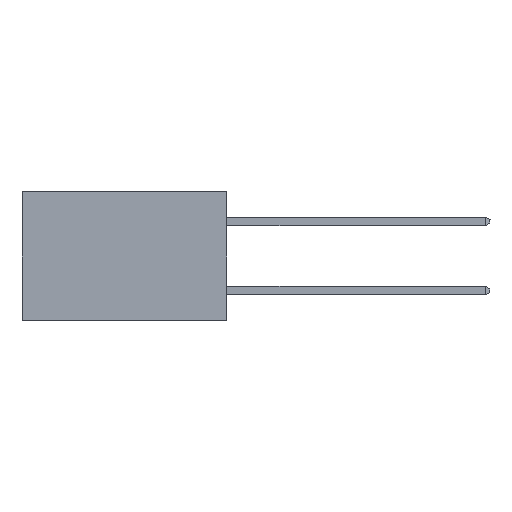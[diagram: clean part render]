
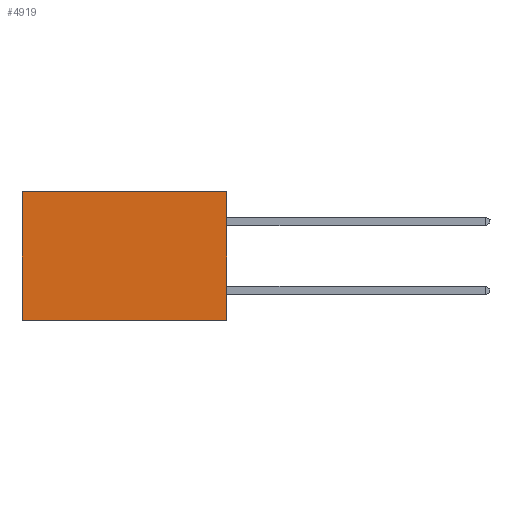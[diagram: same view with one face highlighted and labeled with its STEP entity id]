
A CAD part, left-side view. The second image highlights one B-rep face of the part: STEP entity #4919.
In plain terms, the highlighted planar face has unit normal (-1, 0, 0).
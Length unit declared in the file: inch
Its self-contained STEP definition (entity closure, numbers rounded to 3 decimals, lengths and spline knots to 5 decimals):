
#410 = VECTOR ( 'NONE', #22200, 39.37008 ) ;
#917 = ORIENTED_EDGE ( 'NONE', *, *, #23986, .T. ) ;
#2059 = VECTOR ( 'NONE', #22672, 39.37008 ) ;
#3909 = ORIENTED_EDGE ( 'NONE', *, *, #14130, .F. ) ;
#4919 = ADVANCED_FACE ( 'NONE', ( #15475 ), #14348, .F. ) ;
#5017 = LINE ( 'NONE', #8824, #410 ) ;
#6903 = DIRECTION ( 'NONE',  ( 0., 1., 0. ) ) ;
#8143 = VERTEX_POINT ( 'NONE', #18027 ) ;
#8751 = EDGE_CURVE ( 'NONE', #8143, #22815, #14476, .T. ) ;
#8824 = CARTESIAN_POINT ( 'NONE',  ( 0.277, 0.59, -0.37 ) ) ;
#9307 = VECTOR ( 'NONE', #23433, 39.37008 ) ;
#9668 = EDGE_CURVE ( 'NONE', #15816, #21993, #19501, .T. ) ;
#11166 = EDGE_LOOP ( 'NONE', ( #917, #11948, #3909, #24839 ) ) ;
#11948 = ORIENTED_EDGE ( 'NONE', *, *, #9668, .F. ) ;
#12706 = CARTESIAN_POINT ( 'NONE',  ( 0.277, 0., -0.37 ) ) ;
#12944 = AXIS2_PLACEMENT_3D ( 'NONE', #13612, #13324, #13297 ) ;
#13297 = DIRECTION ( 'NONE',  ( 0., 0., -1. ) ) ;
#13324 = DIRECTION ( 'NONE',  ( 1., 0., 0. ) ) ;
#13612 = CARTESIAN_POINT ( 'NONE',  ( 0.277, 0., -0.37 ) ) ;
#14130 = EDGE_CURVE ( 'NONE', #8143, #15816, #21454, .T. ) ;
#14348 = PLANE ( 'NONE',  #12944 ) ;
#14476 = LINE ( 'NONE', #21560, #9307 ) ;
#14868 = CARTESIAN_POINT ( 'NONE',  ( 0.277, 0.59, 0. ) ) ;
#15475 = FACE_OUTER_BOUND ( 'NONE', #11166, .T. ) ;
#15816 = VERTEX_POINT ( 'NONE', #15846 ) ;
#15846 = CARTESIAN_POINT ( 'NONE',  ( 0.277, 0., -0.37 ) ) ;
#18027 = CARTESIAN_POINT ( 'NONE',  ( 0.277, 0., 0. ) ) ;
#19501 = LINE ( 'NONE', #12706, #23877 ) ;
#20812 = CARTESIAN_POINT ( 'NONE',  ( 0.277, 0., -0.37 ) ) ;
#21454 = LINE ( 'NONE', #20812, #2059 ) ;
#21560 = CARTESIAN_POINT ( 'NONE',  ( 0.277, 0., 0. ) ) ;
#21993 = VERTEX_POINT ( 'NONE', #24049 ) ;
#22200 = DIRECTION ( 'NONE',  ( 0., 0., -1. ) ) ;
#22672 = DIRECTION ( 'NONE',  ( 0., 0., -1. ) ) ;
#22815 = VERTEX_POINT ( 'NONE', #14868 ) ;
#23433 = DIRECTION ( 'NONE',  ( 0., 1., 0. ) ) ;
#23877 = VECTOR ( 'NONE', #6903, 39.37008 ) ;
#23986 = EDGE_CURVE ( 'NONE', #22815, #21993, #5017, .T. ) ;
#24049 = CARTESIAN_POINT ( 'NONE',  ( 0.277, 0.59, -0.37 ) ) ;
#24839 = ORIENTED_EDGE ( 'NONE', *, *, #8751, .T. ) ;
